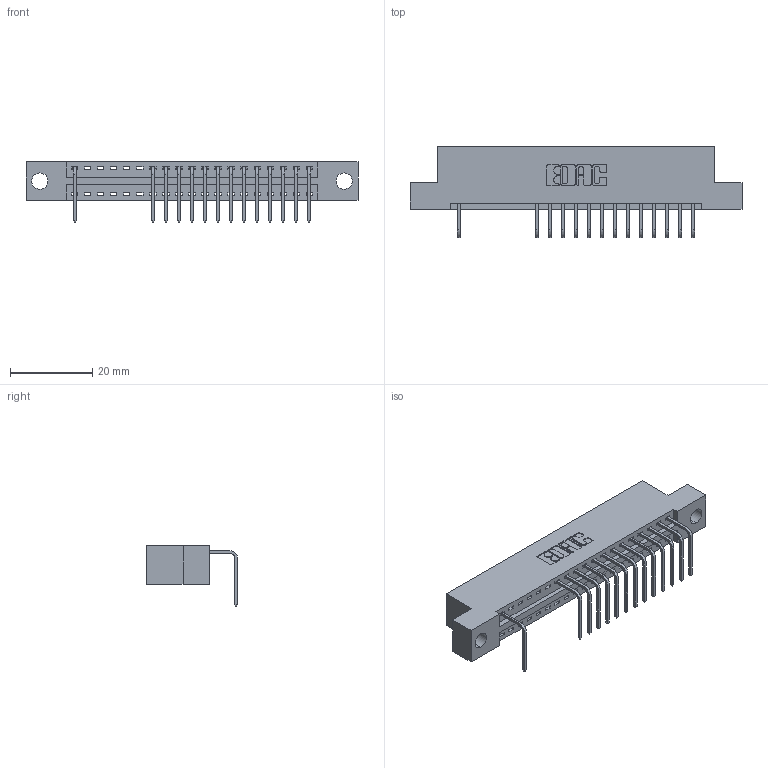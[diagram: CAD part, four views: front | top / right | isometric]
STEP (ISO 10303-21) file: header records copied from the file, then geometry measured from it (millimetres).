
FILE_DESCRIPTION (( 'STEP AP203' ), '1' );
FILE_NAME ('346-019-558-104.STEP', '2018-08-20T10:24:05', ( '' ), ( '' ), 'SwSTEP 2.0', 'SolidWorks 2016', '' );
FILE_SCHEMA (( 'CONFIG_CONTROL_DESIGN' ));
Length unit declared in the file: inch
Products named in the file (3): 346-019-558-104; 346 Part_Flush Mounting Lugs - 0.156 Dia-TH; 345-292-001_558 Tail - 2
Assembly tree (15 placements, depth 2):
  346-019-558-104
    346 Part_Flush Mounting Lugs - 0.156 Dia-TH
    345-292-001_558 Tail - 2  x14
Bounding box: 80.9 x 22.16 x 14.73 mm (x, y, z)
Volume: 7487 mm3; surface area: 8885.1 mm2
Topology: 15 solids, 15 shells, 1022 faces, 3087 edges, 2038 vertices
Faces by surface type: plane 714, cylinder 308
Entity records: 14815 total; most frequent: CARTESIAN_POINT 2576, ORIENTED_EDGE 2534, DIRECTION 2295, EDGE_CURVE 1267, VECTOR 1059, LINE 1059, VERTEX_POINT 842, AXIS2_PLACEMENT_3D 618
